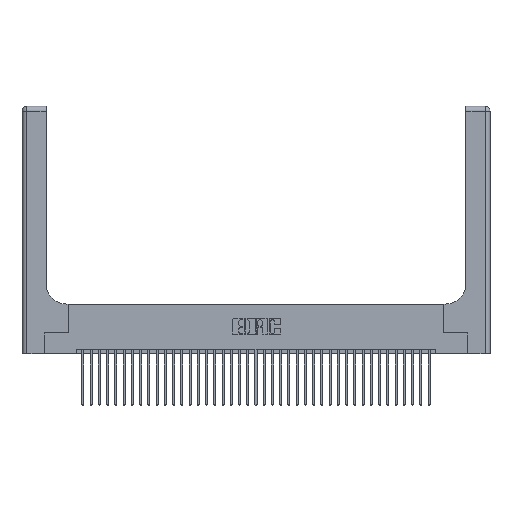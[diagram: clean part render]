
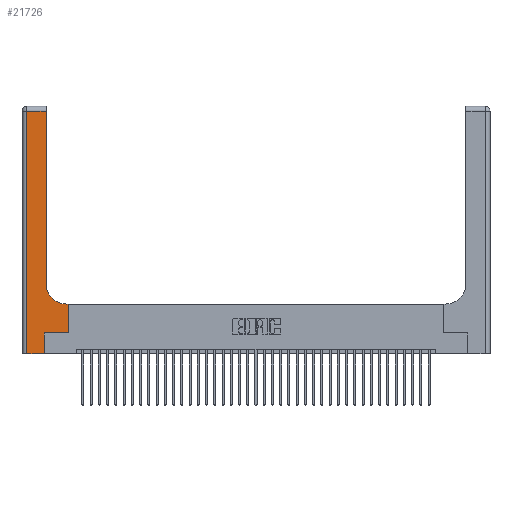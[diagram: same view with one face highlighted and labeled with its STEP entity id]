
A CAD part, top view. The second image highlights one B-rep face of the part: STEP entity #21726.
In plain terms, the highlighted planar face has unit normal (0, 0, 1).
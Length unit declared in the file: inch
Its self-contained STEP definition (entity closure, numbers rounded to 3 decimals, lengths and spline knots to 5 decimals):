
#772 = EDGE_CURVE ( 'NONE', #12832, #12155, #4894, .T. ) ;
#777 = DIRECTION ( 'NONE',  ( 0., 1., 0. ) ) ;
#782 = ORIENTED_EDGE ( 'NONE', *, *, #2156, .T. ) ;
#917 = LINE ( 'NONE', #17494, #28075 ) ;
#1151 = FACE_OUTER_BOUND ( 'NONE', #13325, .T. ) ;
#1547 = ORIENTED_EDGE ( 'NONE', *, *, #2264, .T. ) ;
#1584 = ORIENTED_EDGE ( 'NONE', *, *, #29432, .T. ) ;
#1720 = LINE ( 'NONE', #32890, #34096 ) ;
#1826 = CIRCLE ( 'NONE', #23977, 0.25 ) ;
#2021 = VECTOR ( 'NONE', #7720, 39.37008 ) ;
#2156 = EDGE_CURVE ( 'NONE', #34256, #12832, #25455, .T. ) ;
#2248 = VERTEX_POINT ( 'NONE', #20192 ) ;
#2264 = EDGE_CURVE ( 'NONE', #12155, #3371, #2524, .T. ) ;
#2524 = LINE ( 'NONE', #21601, #2978 ) ;
#2978 = VECTOR ( 'NONE', #22230, 39.37008 ) ;
#2997 = CARTESIAN_POINT ( 'NONE',  ( 0.269, 0., 0.37 ) ) ;
#3015 = DIRECTION ( 'NONE',  ( 1., 0., 0. ) ) ;
#3371 = VERTEX_POINT ( 'NONE', #35690 ) ;
#3737 = VERTEX_POINT ( 'NONE', #22668 ) ;
#4894 = LINE ( 'NONE', #24754, #15206 ) ;
#5645 = VERTEX_POINT ( 'NONE', #7143 ) ;
#6243 = EDGE_CURVE ( 'NONE', #5645, #3737, #18559, .T. ) ;
#6479 = VECTOR ( 'NONE', #24090, 39.37008 ) ;
#7143 = CARTESIAN_POINT ( 'NONE',  ( 0.06, 2.94, 0.37 ) ) ;
#7720 = DIRECTION ( 'NONE',  ( 1., 0., 0. ) ) ;
#10805 = EDGE_CURVE ( 'NONE', #3737, #35553, #1720, .T. ) ;
#12155 = VERTEX_POINT ( 'NONE', #37788 ) ;
#12830 = CARTESIAN_POINT ( 'NONE',  ( 0.06, 3., 0.37 ) ) ;
#12832 = VERTEX_POINT ( 'NONE', #25970 ) ;
#13325 = EDGE_LOOP ( 'NONE', ( #27299, #33311, #29112, #28497, #1584, #782, #33356, #1547, #32348 ) ) ;
#14166 = VERTEX_POINT ( 'NONE', #30024 ) ;
#15206 = VECTOR ( 'NONE', #777, 39.37008 ) ;
#15323 = CARTESIAN_POINT ( 'NONE',  ( 0., 2.94, 0.37 ) ) ;
#16369 = DIRECTION ( 'NONE',  ( 0., 0., -1. ) ) ;
#17324 = DIRECTION ( 'NONE',  ( 0., 1., 0. ) ) ;
#17494 = CARTESIAN_POINT ( 'NONE',  ( 0.2915, 3., 0.37 ) ) ;
#18559 = LINE ( 'NONE', #12830, #28944 ) ;
#18592 = CARTESIAN_POINT ( 'NONE',  ( 0., 3., 0.37 ) ) ;
#20192 = CARTESIAN_POINT ( 'NONE',  ( 0.2915, 2.94, 0.37 ) ) ;
#20526 = VECTOR ( 'NONE', #17324, 39.37008 ) ;
#21495 = LINE ( 'NONE', #15323, #6479 ) ;
#21601 = CARTESIAN_POINT ( 'NONE',  ( 0.2915, 0.6, 0.37 ) ) ;
#21726 = ADVANCED_FACE ( 'NONE', ( #1151 ), #36613, .F. ) ;
#22230 = DIRECTION ( 'NONE',  ( -1., 0., 0. ) ) ;
#22367 = CARTESIAN_POINT ( 'NONE',  ( 0.269, 0.25, 0.37 ) ) ;
#22668 = CARTESIAN_POINT ( 'NONE',  ( 0.06, 0., 0.37 ) ) ;
#22851 = AXIS2_PLACEMENT_3D ( 'NONE', #18592, #24667, #33729 ) ;
#23977 = AXIS2_PLACEMENT_3D ( 'NONE', #25308, #16369, #28325 ) ;
#24090 = DIRECTION ( 'NONE',  ( -1., 0., 0. ) ) ;
#24334 = CARTESIAN_POINT ( 'NONE',  ( 0.269, 0.25, 0.37 ) ) ;
#24667 = DIRECTION ( 'NONE',  ( 0., 0., -1. ) ) ;
#24754 = CARTESIAN_POINT ( 'NONE',  ( 0.5585, 0.25, 0.37 ) ) ;
#25189 = EDGE_CURVE ( 'NONE', #2248, #5645, #21495, .T. ) ;
#25308 = CARTESIAN_POINT ( 'NONE',  ( 0.5415, 0.85, 0.37 ) ) ;
#25455 = LINE ( 'NONE', #22367, #2021 ) ;
#25659 = EDGE_CURVE ( 'NONE', #3371, #14166, #1826, .T. ) ;
#25970 = CARTESIAN_POINT ( 'NONE',  ( 0.5585, 0.25, 0.37 ) ) ;
#27299 = ORIENTED_EDGE ( 'NONE', *, *, #30732, .T. ) ;
#28075 = VECTOR ( 'NONE', #29636, 39.37008 ) ;
#28325 = DIRECTION ( 'NONE',  ( 1., 0., 0. ) ) ;
#28497 = ORIENTED_EDGE ( 'NONE', *, *, #10805, .T. ) ;
#28944 = VECTOR ( 'NONE', #33838, 39.37008 ) ;
#29112 = ORIENTED_EDGE ( 'NONE', *, *, #6243, .T. ) ;
#29327 = CARTESIAN_POINT ( 'NONE',  ( 0.269, 0., 0.37 ) ) ;
#29432 = EDGE_CURVE ( 'NONE', #35553, #34256, #34201, .T. ) ;
#29636 = DIRECTION ( 'NONE',  ( 0., 1., 0. ) ) ;
#30024 = CARTESIAN_POINT ( 'NONE',  ( 0.2915, 0.85, 0.37 ) ) ;
#30732 = EDGE_CURVE ( 'NONE', #14166, #2248, #917, .T. ) ;
#32348 = ORIENTED_EDGE ( 'NONE', *, *, #25659, .T. ) ;
#32890 = CARTESIAN_POINT ( 'NONE',  ( 0., 0., 0.37 ) ) ;
#33311 = ORIENTED_EDGE ( 'NONE', *, *, #25189, .T. ) ;
#33356 = ORIENTED_EDGE ( 'NONE', *, *, #772, .T. ) ;
#33729 = DIRECTION ( 'NONE',  ( -1., 0., 0. ) ) ;
#33838 = DIRECTION ( 'NONE',  ( 0., -1., 0. ) ) ;
#34096 = VECTOR ( 'NONE', #3015, 39.37008 ) ;
#34201 = LINE ( 'NONE', #2997, #20526 ) ;
#34256 = VERTEX_POINT ( 'NONE', #24334 ) ;
#35553 = VERTEX_POINT ( 'NONE', #29327 ) ;
#35690 = CARTESIAN_POINT ( 'NONE',  ( 0.5415, 0.6, 0.37 ) ) ;
#36613 = PLANE ( 'NONE',  #22851 ) ;
#37788 = CARTESIAN_POINT ( 'NONE',  ( 0.5585, 0.6, 0.37 ) ) ;
